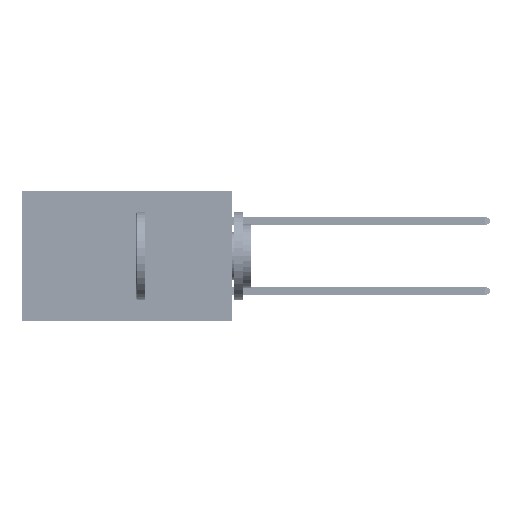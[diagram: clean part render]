
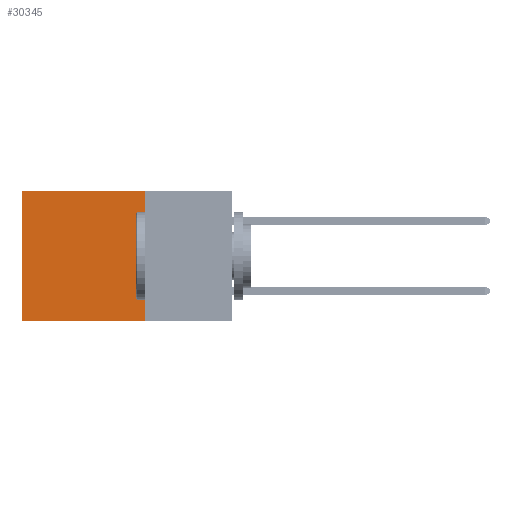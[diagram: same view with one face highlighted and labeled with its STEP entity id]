
A CAD part, left-side view. The second image highlights one B-rep face of the part: STEP entity #30345.
In plain terms, the highlighted planar face has unit normal (-1, 0, 0).
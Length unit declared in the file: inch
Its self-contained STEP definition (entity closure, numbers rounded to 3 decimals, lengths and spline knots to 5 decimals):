
#223 = PLANE ( 'NONE',  #20765 ) ;
#1994 = CARTESIAN_POINT ( 'NONE',  ( 0.2875, 0.25, 0. ) ) ;
#2340 = FACE_OUTER_BOUND ( 'NONE', #21228, .T. ) ;
#3098 = VECTOR ( 'NONE', #34005, 39.37008 ) ;
#3945 = ORIENTED_EDGE ( 'NONE', *, *, #28553, .T. ) ;
#4372 = LINE ( 'NONE', #30216, #3098 ) ;
#7657 = CARTESIAN_POINT ( 'NONE',  ( 0.2875, 0.25, -0.37 ) ) ;
#8433 = VERTEX_POINT ( 'NONE', #36451 ) ;
#9539 = VECTOR ( 'NONE', #31644, 39.37008 ) ;
#10564 = CARTESIAN_POINT ( 'NONE',  ( 0.2875, 0.25, -0.37 ) ) ;
#10843 = LINE ( 'NONE', #27673, #9539 ) ;
#13226 = CARTESIAN_POINT ( 'NONE',  ( 0.2875, 0.25, 0. ) ) ;
#14081 = ORIENTED_EDGE ( 'NONE', *, *, #45906, .F. ) ;
#14251 = VECTOR ( 'NONE', #51471, 39.37008 ) ;
#15036 = VERTEX_POINT ( 'NONE', #47208 ) ;
#17343 = DIRECTION ( 'NONE',  ( 0., 0., -1. ) ) ;
#17632 = VERTEX_POINT ( 'NONE', #39772 ) ;
#20765 = AXIS2_PLACEMENT_3D ( 'NONE', #13226, #41106, #17343 ) ;
#21228 = EDGE_LOOP ( 'NONE', ( #42833, #14081, #42520, #3945 ) ) ;
#24366 = EDGE_CURVE ( 'NONE', #8433, #15036, #10843, .T. ) ;
#25842 = EDGE_CURVE ( 'NONE', #17632, #30015, #44333, .T. ) ;
#26206 = DIRECTION ( 'NONE',  ( 0., 0., -1. ) ) ;
#27447 = LINE ( 'NONE', #7657, #14251 ) ;
#27673 = CARTESIAN_POINT ( 'NONE',  ( 0.2875, 0.6, 0. ) ) ;
#28553 = EDGE_CURVE ( 'NONE', #17632, #8433, #4372, .T. ) ;
#30015 = VERTEX_POINT ( 'NONE', #10564 ) ;
#30216 = CARTESIAN_POINT ( 'NONE',  ( 0.2875, 0.25, 0. ) ) ;
#30345 = ADVANCED_FACE ( 'NONE', ( #2340 ), #223, .F. ) ;
#31644 = DIRECTION ( 'NONE',  ( 0., 0., -1. ) ) ;
#34005 = DIRECTION ( 'NONE',  ( 0., 1., 0. ) ) ;
#35114 = VECTOR ( 'NONE', #26206, 39.37008 ) ;
#36451 = CARTESIAN_POINT ( 'NONE',  ( 0.2875, 0.6, 0. ) ) ;
#39772 = CARTESIAN_POINT ( 'NONE',  ( 0.2875, 0.25, 0. ) ) ;
#41106 = DIRECTION ( 'NONE',  ( 1., 0., 0. ) ) ;
#42520 = ORIENTED_EDGE ( 'NONE', *, *, #25842, .F. ) ;
#42833 = ORIENTED_EDGE ( 'NONE', *, *, #24366, .T. ) ;
#44333 = LINE ( 'NONE', #1994, #35114 ) ;
#45906 = EDGE_CURVE ( 'NONE', #30015, #15036, #27447, .T. ) ;
#47208 = CARTESIAN_POINT ( 'NONE',  ( 0.2875, 0.6, -0.37 ) ) ;
#51471 = DIRECTION ( 'NONE',  ( 0., 1., 0. ) ) ;
